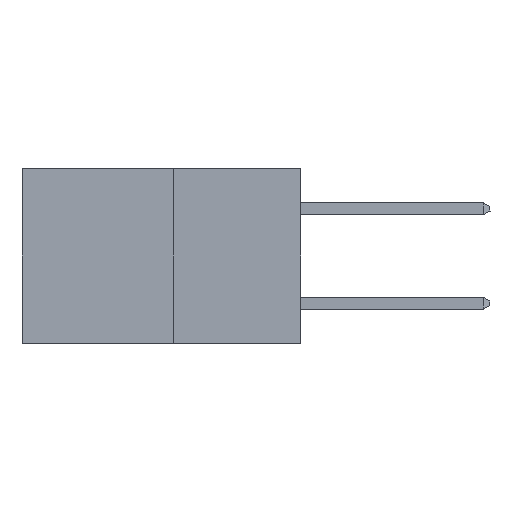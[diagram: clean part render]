
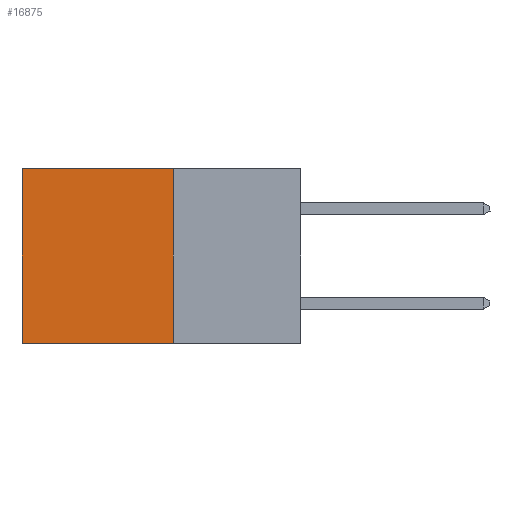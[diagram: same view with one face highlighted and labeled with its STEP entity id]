
A CAD part, left-side view. The second image highlights one B-rep face of the part: STEP entity #16875.
In plain terms, the highlighted planar face has unit normal (-1, 0, 0).
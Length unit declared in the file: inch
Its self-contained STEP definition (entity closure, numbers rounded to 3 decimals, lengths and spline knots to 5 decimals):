
#570 = FACE_OUTER_BOUND ( 'NONE', #2112, .T. ) ;
#1093 = CARTESIAN_POINT ( 'NONE',  ( 0.277, 0.27, -0.37 ) ) ;
#2112 = EDGE_LOOP ( 'NONE', ( #14030, #7478, #11258, #19095 ) ) ;
#2321 = VECTOR ( 'NONE', #7083, 39.37008 ) ;
#2663 = EDGE_CURVE ( 'NONE', #9493, #14702, #16246, .T. ) ;
#2698 = DIRECTION ( 'NONE',  ( 1., 0., 0. ) ) ;
#3138 = EDGE_CURVE ( 'NONE', #13568, #12623, #16675, .T. ) ;
#3236 = CARTESIAN_POINT ( 'NONE',  ( 0.277, 0.59, 0. ) ) ;
#3470 = DIRECTION ( 'NONE',  ( 0., 1., 0. ) ) ;
#3532 = CARTESIAN_POINT ( 'NONE',  ( 0.277, 0.27, -0.37 ) ) ;
#3888 = AXIS2_PLACEMENT_3D ( 'NONE', #16177, #2698, #13266 ) ;
#4056 = CARTESIAN_POINT ( 'NONE',  ( 0.277, 0.27, -0.37 ) ) ;
#4296 = VECTOR ( 'NONE', #4373, 39.37008 ) ;
#4373 = DIRECTION ( 'NONE',  ( 0., 0., -1. ) ) ;
#4611 = CARTESIAN_POINT ( 'NONE',  ( 0.277, 0.59, -0.37 ) ) ;
#5010 = DIRECTION ( 'NONE',  ( 0., 0., -1. ) ) ;
#5691 = EDGE_CURVE ( 'NONE', #12623, #14702, #16606, .T. ) ;
#6067 = CARTESIAN_POINT ( 'NONE',  ( 0.277, 0.59, -0.37 ) ) ;
#7083 = DIRECTION ( 'NONE',  ( 0., 1., 0. ) ) ;
#7478 = ORIENTED_EDGE ( 'NONE', *, *, #5691, .F. ) ;
#8292 = VECTOR ( 'NONE', #5010, 39.37008 ) ;
#9493 = VERTEX_POINT ( 'NONE', #3236 ) ;
#10262 = PLANE ( 'NONE',  #3888 ) ;
#11258 = ORIENTED_EDGE ( 'NONE', *, *, #3138, .F. ) ;
#12239 = VECTOR ( 'NONE', #3470, 39.37008 ) ;
#12623 = VERTEX_POINT ( 'NONE', #1093 ) ;
#13266 = DIRECTION ( 'NONE',  ( 0., 0., -1. ) ) ;
#13568 = VERTEX_POINT ( 'NONE', #18129 ) ;
#14030 = ORIENTED_EDGE ( 'NONE', *, *, #2663, .T. ) ;
#14702 = VERTEX_POINT ( 'NONE', #6067 ) ;
#16015 = CARTESIAN_POINT ( 'NONE',  ( 0.277, 0.27, 0. ) ) ;
#16108 = EDGE_CURVE ( 'NONE', #13568, #9493, #17757, .T. ) ;
#16177 = CARTESIAN_POINT ( 'NONE',  ( 0.277, 0.27, -0.37 ) ) ;
#16246 = LINE ( 'NONE', #4611, #4296 ) ;
#16606 = LINE ( 'NONE', #3532, #12239 ) ;
#16675 = LINE ( 'NONE', #4056, #8292 ) ;
#16875 = ADVANCED_FACE ( 'NONE', ( #570 ), #10262, .F. ) ;
#17757 = LINE ( 'NONE', #16015, #2321 ) ;
#18129 = CARTESIAN_POINT ( 'NONE',  ( 0.277, 0.27, 0. ) ) ;
#19095 = ORIENTED_EDGE ( 'NONE', *, *, #16108, .T. ) ;
